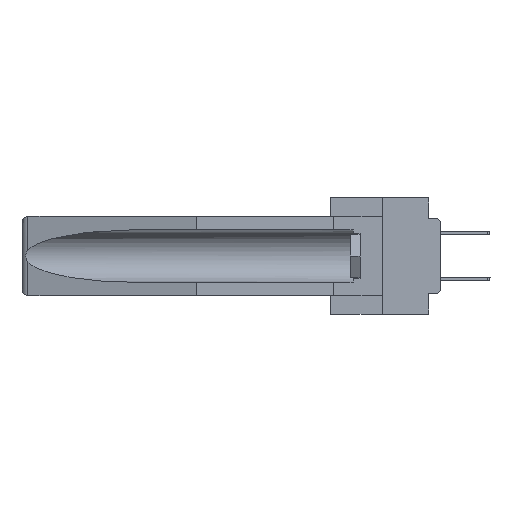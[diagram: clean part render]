
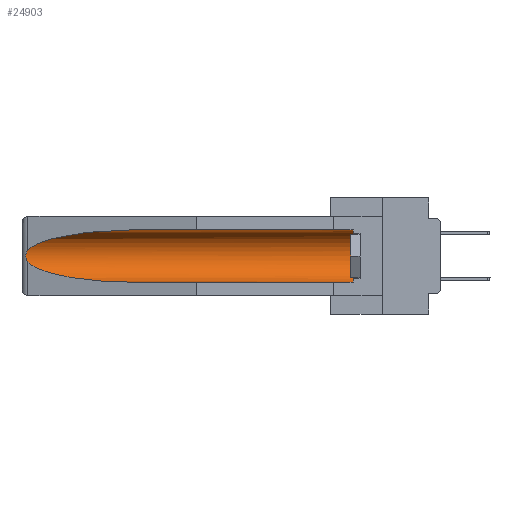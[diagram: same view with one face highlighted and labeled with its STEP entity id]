
A CAD part, left-side view. The second image highlights one B-rep face of the part: STEP entity #24903.
In plain terms, the highlighted cylindrical face has radius 2.857 mm (diameter 5.715 mm), a partial arc.
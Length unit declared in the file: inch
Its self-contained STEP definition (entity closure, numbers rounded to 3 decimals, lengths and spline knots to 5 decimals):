
#1346 = DIRECTION ( 'NONE',  ( 0., 1., 0. ) ) ;
#1617 = CARTESIAN_POINT ( 'NONE',  ( 0.155, 1.07973, -0.059 ) ) ;
#1629 = CARTESIAN_POINT ( 'NONE',  ( 0.155, 1.07973, -0.284 ) ) ;
#1711 = VERTEX_POINT ( 'NONE', #33270 ) ;
#1900 = EDGE_CURVE ( 'NONE', #19447, #31780, #7415, .T. ) ;
#1944 = CARTESIAN_POINT ( 'NONE',  ( 0.155, -0.30754, -0.059 ) ) ;
#2029 = CARTESIAN_POINT ( 'NONE',  ( 0.21114, 1.30732, -0.284 ) ) ;
#2417 = DIRECTION ( 'NONE',  ( 0., 0., 1. ) ) ;
#2466 = DIRECTION ( 'NONE',  ( 0., -1., 0. ) ) ;
#3201 = CARTESIAN_POINT ( 'NONE',  ( 0.26537, 1.52718, -0.19328 ) ) ;
#3504 = CARTESIAN_POINT ( 'NONE',  ( 0.155, -0.30754, -0.1715 ) ) ;
#4115 = DIRECTION ( 'NONE',  ( 0., 1., 0. ) ) ;
#4995 = CARTESIAN_POINT ( 'NONE',  ( 0.26655, 1.53094, -0.18657 ) ) ;
#5374 = CARTESIAN_POINT ( 'NONE',  ( 0.2673, 1.53269, -0.17917 ) ) ;
#5428 = CARTESIAN_POINT ( 'NONE',  ( 0.155, 0.126, -0.1715 ) ) ;
#6418 = CARTESIAN_POINT ( 'NONE',  ( 0.155, 1.07973, -0.284 ) ) ;
#7415 =( BOUNDED_CURVE ( )  B_SPLINE_CURVE ( 3, ( #19829, #37593, #2029, #1629 ),
 .UNSPECIFIED., .F., .F. ) 
 B_SPLINE_CURVE_WITH_KNOTS ( ( 4, 4 ),
 ( 0.1948, 1.5708 ),
 .UNSPECIFIED. ) 
 CURVE ( )  GEOMETRIC_REPRESENTATION_ITEM ( )  RATIONAL_B_SPLINE_CURVE ( ( 1., 0.848, 0.848, 1. ) ) 
 REPRESENTATION_ITEM ( '' )  );
#8251 = CARTESIAN_POINT ( 'NONE',  ( 0.155, 0.126, -0.059 ) ) ;
#8519 = CARTESIAN_POINT ( 'NONE',  ( 0.26537, 1.52718, -0.19328 ) ) ;
#11109 = CARTESIAN_POINT ( 'NONE',  ( 0.26597, 1.52961, -0.15275 ) ) ;
#12017 = DIRECTION ( 'NONE',  ( 0., 0., 1. ) ) ;
#13657 = ORIENTED_EDGE ( 'NONE', *, *, #36349, .T. ) ;
#13891 = CARTESIAN_POINT ( 'NONE',  ( 0.26537, 1.52718, -0.14972 ) ) ;
#14262 = CARTESIAN_POINT ( 'NONE',  ( 0.26597, 1.5296, -0.19026 ) ) ;
#15126 = EDGE_CURVE ( 'NONE', #17017, #20972, #29035, .T. ) ;
#15762 = AXIS2_PLACEMENT_3D ( 'NONE', #5428, #2466, #2417 ) ;
#17017 = VERTEX_POINT ( 'NONE', #8251 ) ;
#17641 = ORIENTED_EDGE ( 'NONE', *, *, #35212, .F. ) ;
#17701 = CARTESIAN_POINT ( 'NONE',  ( 0.155, 1.07973, -0.059 ) ) ;
#18447 = ORIENTED_EDGE ( 'NONE', *, *, #1900, .T. ) ;
#19447 = VERTEX_POINT ( 'NONE', #3201 ) ;
#19829 = CARTESIAN_POINT ( 'NONE',  ( 0.26537, 1.52718, -0.19328 ) ) ;
#20213 = CARTESIAN_POINT ( 'NONE',  ( 0.2673, 1.5327, -0.16383 ) ) ;
#20972 = VERTEX_POINT ( 'NONE', #17701 ) ;
#21322 = ORIENTED_EDGE ( 'NONE', *, *, #32326, .T. ) ;
#21584 = EDGE_LOOP ( 'NONE', ( #21322, #13657, #18447, #17641, #24148, #24917 ) ) ;
#22477 = LINE ( 'NONE', #25848, #30834 ) ;
#23874 = CARTESIAN_POINT ( 'NONE',  ( 0.26537, 1.52718, -0.14972 ) ) ;
#24075 = VECTOR ( 'NONE', #4115, 39.37008 ) ;
#24148 = ORIENTED_EDGE ( 'NONE', *, *, #37307, .T. ) ;
#24656 = CYLINDRICAL_SURFACE ( 'NONE', #33362, 0.1125 ) ;
#24903 = ADVANCED_FACE ( 'NONE', ( #30608 ), #24656, .F. ) ;
#24917 = ORIENTED_EDGE ( 'NONE', *, *, #15126, .T. ) ;
#25649 =( BOUNDED_CURVE ( )  B_SPLINE_CURVE ( 3, ( #1617, #37401, #31694, #25736 ),
 .UNSPECIFIED., .F., .F. ) 
 B_SPLINE_CURVE_WITH_KNOTS ( ( 4, 4 ),
 ( 4.71239, 6.08839 ),
 .UNSPECIFIED. ) 
 CURVE ( )  GEOMETRIC_REPRESENTATION_ITEM ( )  RATIONAL_B_SPLINE_CURVE ( ( 1., 0.848, 0.848, 1. ) ) 
 REPRESENTATION_ITEM ( '' )  );
#25736 = CARTESIAN_POINT ( 'NONE',  ( 0.26537, 1.52718, -0.14972 ) ) ;
#25848 = CARTESIAN_POINT ( 'NONE',  ( 0.155, -0.30754, -0.284 ) ) ;
#28852 = B_SPLINE_CURVE_WITH_KNOTS ( 'NONE', 3,
 ( #13891, #11109, #35035, #20213, #34848, #38568, #5374, #4995, #14262, #8519 ),
 .UNSPECIFIED., .F., .F.,
 ( 4, 2, 2, 2, 4 ),
 ( 0., 0.00029, 0.00058, 0.00087, 0.00117 ),
 .UNSPECIFIED. ) ;
#29035 = LINE ( 'NONE', #1944, #24075 ) ;
#30608 = FACE_OUTER_BOUND ( 'NONE', #21584, .T. ) ;
#30834 = VECTOR ( 'NONE', #1346, 39.37008 ) ;
#31564 = CIRCLE ( 'NONE', #15762, 0.1125 ) ;
#31694 = CARTESIAN_POINT ( 'NONE',  ( 0.25451, 1.48313, -0.09465 ) ) ;
#31780 = VERTEX_POINT ( 'NONE', #6418 ) ;
#32326 = EDGE_CURVE ( 'NONE', #20972, #33709, #25649, .T. ) ;
#33270 = CARTESIAN_POINT ( 'NONE',  ( 0.155, 0.126, -0.284 ) ) ;
#33362 = AXIS2_PLACEMENT_3D ( 'NONE', #3504, #36298, #12017 ) ;
#33709 = VERTEX_POINT ( 'NONE', #23874 ) ;
#34848 = CARTESIAN_POINT ( 'NONE',  ( 0.2675, 1.53308, -0.16763 ) ) ;
#35035 = CARTESIAN_POINT ( 'NONE',  ( 0.26654, 1.53092, -0.15636 ) ) ;
#35212 = EDGE_CURVE ( 'NONE', #1711, #31780, #22477, .T. ) ;
#36298 = DIRECTION ( 'NONE',  ( 0., 1., 0. ) ) ;
#36349 = EDGE_CURVE ( 'NONE', #33709, #19447, #28852, .T. ) ;
#37307 = EDGE_CURVE ( 'NONE', #1711, #17017, #31564, .T. ) ;
#37401 = CARTESIAN_POINT ( 'NONE',  ( 0.21114, 1.30732, -0.059 ) ) ;
#37593 = CARTESIAN_POINT ( 'NONE',  ( 0.25451, 1.48313, -0.24835 ) ) ;
#38568 = CARTESIAN_POINT ( 'NONE',  ( 0.2675, 1.53308, -0.17534 ) ) ;
